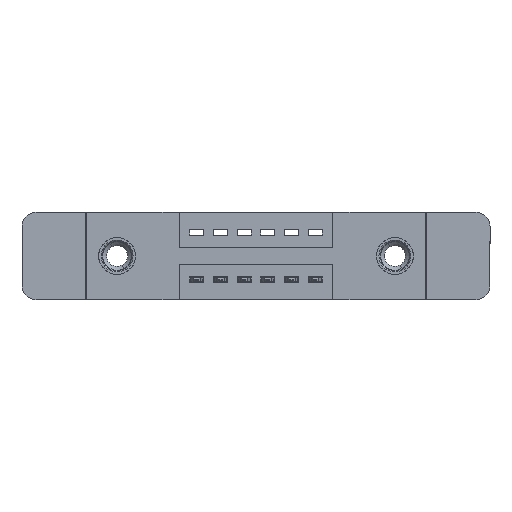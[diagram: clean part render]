
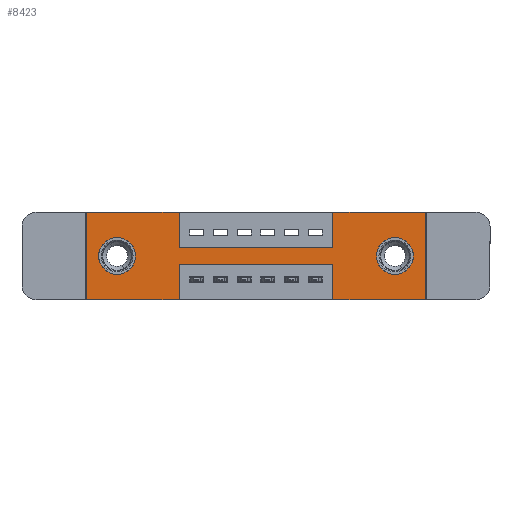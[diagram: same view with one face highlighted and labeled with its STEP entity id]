
A CAD part, front view. The second image highlights one B-rep face of the part: STEP entity #8423.
In plain terms, the highlighted planar face has unit normal (0, -1, 0).
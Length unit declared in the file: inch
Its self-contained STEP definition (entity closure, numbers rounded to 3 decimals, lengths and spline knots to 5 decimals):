
#94 = VERTEX_POINT ( 'NONE', #1673 ) ;
#147 = VERTEX_POINT ( 'NONE', #4214 ) ;
#158 = LINE ( 'NONE', #1594, #10441 ) ;
#370 = CARTESIAN_POINT ( 'NONE',  ( 1.305, 0., -0.185 ) ) ;
#415 = EDGE_CURVE ( 'NONE', #94, #5725, #7992, .T. ) ;
#497 = EDGE_LOOP ( 'NONE', ( #1147, #8711 ) ) ;
#560 = DIRECTION ( 'NONE',  ( 0., 0., -1. ) ) ;
#591 = DIRECTION ( 'NONE',  ( 0., 0., -1. ) ) ;
#706 = EDGE_CURVE ( 'NONE', #5725, #1700, #8682, .T. ) ;
#712 = PLANE ( 'NONE',  #7056 ) ;
#875 = VERTEX_POINT ( 'NONE', #2429 ) ;
#1141 = EDGE_CURVE ( 'NONE', #4067, #6682, #10605, .T. ) ;
#1147 = ORIENTED_EDGE ( 'NONE', *, *, #10740, .T. ) ;
#1435 = LINE ( 'NONE', #14208, #4059 ) ;
#1502 = ORIENTED_EDGE ( 'NONE', *, *, #9328, .F. ) ;
#1551 = DIRECTION ( 'NONE',  ( 0., 0., -1. ) ) ;
#1594 = CARTESIAN_POINT ( 'NONE',  ( 0.3925, 0., 0. ) ) ;
#1625 = EDGE_LOOP ( 'NONE', ( #4942, #13514, #14513, #9160, #2461, #1502, #2628, #13078, #1680, #3032, #5170, #10552 ) ) ;
#1673 = CARTESIAN_POINT ( 'NONE',  ( 1.435, 0., 0. ) ) ;
#1680 = ORIENTED_EDGE ( 'NONE', *, *, #2810, .F. ) ;
#1700 = VERTEX_POINT ( 'NONE', #3215 ) ;
#2200 = VERTEX_POINT ( 'NONE', #8379 ) ;
#2230 = EDGE_CURVE ( 'NONE', #14112, #12420, #10853, .T. ) ;
#2241 = DIRECTION ( 'NONE',  ( -1., 0., 0. ) ) ;
#2372 = AXIS2_PLACEMENT_3D ( 'NONE', #2486, #11525, #8225 ) ;
#2402 = EDGE_LOOP ( 'NONE', ( #5447, #10381 ) ) ;
#2429 = CARTESIAN_POINT ( 'NONE',  ( 0.13, 0., -0.107 ) ) ;
#2461 = ORIENTED_EDGE ( 'NONE', *, *, #415, .F. ) ;
#2466 = LINE ( 'NONE', #12484, #8844 ) ;
#2486 = CARTESIAN_POINT ( 'NONE',  ( 0.13, 0., -0.185 ) ) ;
#2627 = DIRECTION ( 'NONE',  ( 0., 0., -1. ) ) ;
#2628 = ORIENTED_EDGE ( 'NONE', *, *, #3161, .F. ) ;
#2651 = DIRECTION ( 'NONE',  ( -1., 0., 0. ) ) ;
#2701 = VERTEX_POINT ( 'NONE', #5728 ) ;
#2810 = EDGE_CURVE ( 'NONE', #6682, #5555, #158, .T. ) ;
#3032 = ORIENTED_EDGE ( 'NONE', *, *, #1141, .F. ) ;
#3161 = EDGE_CURVE ( 'NONE', #147, #13618, #6078, .T. ) ;
#3215 = CARTESIAN_POINT ( 'NONE',  ( 1.0425, 0., -0.37 ) ) ;
#3290 = AXIS2_PLACEMENT_3D ( 'NONE', #6904, #9589, #4974 ) ;
#3396 = VECTOR ( 'NONE', #10511, 39.37008 ) ;
#3418 = EDGE_CURVE ( 'NONE', #14611, #11170, #12412, .T. ) ;
#3650 = VECTOR ( 'NONE', #12302, 39.37008 ) ;
#4014 = LINE ( 'NONE', #13456, #3650 ) ;
#4059 = VECTOR ( 'NONE', #10851, 39.37008 ) ;
#4067 = VERTEX_POINT ( 'NONE', #6693 ) ;
#4214 = CARTESIAN_POINT ( 'NONE',  ( 1.0425, 0., -0.15 ) ) ;
#4367 = CARTESIAN_POINT ( 'NONE',  ( 0.3925, 0., -0.37 ) ) ;
#4815 = LINE ( 'NONE', #4888, #3396 ) ;
#4839 = CARTESIAN_POINT ( 'NONE',  ( 0., 0., 0. ) ) ;
#4888 = CARTESIAN_POINT ( 'NONE',  ( 1.0425, 0., -0.37 ) ) ;
#4942 = ORIENTED_EDGE ( 'NONE', *, *, #3418, .F. ) ;
#4974 = DIRECTION ( 'NONE',  ( 0., 0., 1. ) ) ;
#5170 = ORIENTED_EDGE ( 'NONE', *, *, #11163, .F. ) ;
#5447 = ORIENTED_EDGE ( 'NONE', *, *, #6535, .T. ) ;
#5555 = VERTEX_POINT ( 'NONE', #8791 ) ;
#5648 = VECTOR ( 'NONE', #8760, 39.37008 ) ;
#5725 = VERTEX_POINT ( 'NONE', #10052 ) ;
#5728 = CARTESIAN_POINT ( 'NONE',  ( 0., 0., -0.37 ) ) ;
#5973 = DIRECTION ( 'NONE',  ( 1., 0., 0. ) ) ;
#6078 = LINE ( 'NONE', #8991, #11801 ) ;
#6445 = CARTESIAN_POINT ( 'NONE',  ( 0., 0., -0.37 ) ) ;
#6506 = AXIS2_PLACEMENT_3D ( 'NONE', #370, #7164, #1551 ) ;
#6535 = EDGE_CURVE ( 'NONE', #12420, #14112, #7848, .T. ) ;
#6612 = CARTESIAN_POINT ( 'NONE',  ( 0.3925, 0., -0.37 ) ) ;
#6682 = VERTEX_POINT ( 'NONE', #11733 ) ;
#6693 = CARTESIAN_POINT ( 'NONE',  ( 0., 0., 0. ) ) ;
#6904 = CARTESIAN_POINT ( 'NONE',  ( 0.13, 0., -0.185 ) ) ;
#7056 = AXIS2_PLACEMENT_3D ( 'NONE', #7478, #7383, #560 ) ;
#7129 = CARTESIAN_POINT ( 'NONE',  ( 1.305, 0., -0.185 ) ) ;
#7164 = DIRECTION ( 'NONE',  ( 0., 1., 0. ) ) ;
#7276 = FACE_BOUND ( 'NONE', #497, .T. ) ;
#7383 = DIRECTION ( 'NONE',  ( 0., -1., 0. ) ) ;
#7478 = CARTESIAN_POINT ( 'NONE',  ( 0., 0., -0.37 ) ) ;
#7632 = FACE_OUTER_BOUND ( 'NONE', #1625, .T. ) ;
#7716 = DIRECTION ( 'NONE',  ( 0., 0., -1. ) ) ;
#7807 = CARTESIAN_POINT ( 'NONE',  ( 1.0425, 0., -0.22 ) ) ;
#7848 = CIRCLE ( 'NONE', #6506, 0.078 ) ;
#7936 = VECTOR ( 'NONE', #2651, 39.37008 ) ;
#7970 = FACE_BOUND ( 'NONE', #2402, .T. ) ;
#7992 = LINE ( 'NONE', #8221, #8351 ) ;
#8221 = CARTESIAN_POINT ( 'NONE',  ( 1.435, 0., 0. ) ) ;
#8225 = DIRECTION ( 'NONE',  ( 0., 0., 1. ) ) ;
#8262 = DIRECTION ( 'NONE',  ( 1., 0., 0. ) ) ;
#8351 = VECTOR ( 'NONE', #2627, 39.37008 ) ;
#8379 = CARTESIAN_POINT ( 'NONE',  ( 0.13, 0., -0.263 ) ) ;
#8387 = CIRCLE ( 'NONE', #2372, 0.078 ) ;
#8423 = ADVANCED_FACE ( 'NONE', ( #7970, #7276, #7632 ), #712, .T. ) ;
#8682 = LINE ( 'NONE', #6445, #5648 ) ;
#8711 = ORIENTED_EDGE ( 'NONE', *, *, #13481, .T. ) ;
#8760 = DIRECTION ( 'NONE',  ( -1., 0., 0. ) ) ;
#8791 = CARTESIAN_POINT ( 'NONE',  ( 0.3925, 0., -0.15 ) ) ;
#8802 = VECTOR ( 'NONE', #8262, 39.37008 ) ;
#8844 = VECTOR ( 'NONE', #5973, 39.37008 ) ;
#8991 = CARTESIAN_POINT ( 'NONE',  ( 1.0425, 0., 0. ) ) ;
#9091 = DIRECTION ( 'NONE',  ( 0., 0., 1. ) ) ;
#9096 = AXIS2_PLACEMENT_3D ( 'NONE', #7129, #9419, #10636 ) ;
#9148 = EDGE_CURVE ( 'NONE', #5555, #147, #1435, .T. ) ;
#9160 = ORIENTED_EDGE ( 'NONE', *, *, #706, .F. ) ;
#9328 = EDGE_CURVE ( 'NONE', #13618, #94, #2466, .T. ) ;
#9348 = CIRCLE ( 'NONE', #3290, 0.078 ) ;
#9419 = DIRECTION ( 'NONE',  ( 0., 1., 0. ) ) ;
#9589 = DIRECTION ( 'NONE',  ( 0., 1., 0. ) ) ;
#10052 = CARTESIAN_POINT ( 'NONE',  ( 1.435, 0., -0.37 ) ) ;
#10260 = CARTESIAN_POINT ( 'NONE',  ( 0.3925, 0., -0.22 ) ) ;
#10335 = VECTOR ( 'NONE', #2241, 39.37008 ) ;
#10353 = VERTEX_POINT ( 'NONE', #7807 ) ;
#10381 = ORIENTED_EDGE ( 'NONE', *, *, #2230, .T. ) ;
#10441 = VECTOR ( 'NONE', #591, 39.37008 ) ;
#10511 = DIRECTION ( 'NONE',  ( 0., 0., 1. ) ) ;
#10552 = ORIENTED_EDGE ( 'NONE', *, *, #10588, .F. ) ;
#10588 = EDGE_CURVE ( 'NONE', #11170, #2701, #13285, .T. ) ;
#10605 = LINE ( 'NONE', #4839, #8802 ) ;
#10636 = DIRECTION ( 'NONE',  ( 0., 0., -1. ) ) ;
#10740 = EDGE_CURVE ( 'NONE', #875, #2200, #9348, .T. ) ;
#10851 = DIRECTION ( 'NONE',  ( 1., 0., 0. ) ) ;
#10853 = CIRCLE ( 'NONE', #9096, 0.078 ) ;
#11163 = EDGE_CURVE ( 'NONE', #2701, #4067, #4014, .T. ) ;
#11170 = VERTEX_POINT ( 'NONE', #6612 ) ;
#11403 = CARTESIAN_POINT ( 'NONE',  ( 0.3925, 0., -0.22 ) ) ;
#11525 = DIRECTION ( 'NONE',  ( 0., 1., 0. ) ) ;
#11679 = VECTOR ( 'NONE', #7716, 39.37008 ) ;
#11733 = CARTESIAN_POINT ( 'NONE',  ( 0.3925, 0., 0. ) ) ;
#11771 = CARTESIAN_POINT ( 'NONE',  ( 1.305, 0., -0.107 ) ) ;
#11801 = VECTOR ( 'NONE', #9091, 39.37008 ) ;
#12302 = DIRECTION ( 'NONE',  ( 0., 0., 1. ) ) ;
#12412 = LINE ( 'NONE', #4367, #11679 ) ;
#12420 = VERTEX_POINT ( 'NONE', #11771 ) ;
#12484 = CARTESIAN_POINT ( 'NONE',  ( 0., 0., 0. ) ) ;
#12740 = CARTESIAN_POINT ( 'NONE',  ( 0., 0., -0.37 ) ) ;
#12905 = CARTESIAN_POINT ( 'NONE',  ( 1.305, 0., -0.263 ) ) ;
#13078 = ORIENTED_EDGE ( 'NONE', *, *, #9148, .F. ) ;
#13175 = LINE ( 'NONE', #10260, #10335 ) ;
#13285 = LINE ( 'NONE', #12740, #7936 ) ;
#13456 = CARTESIAN_POINT ( 'NONE',  ( 0., 0., 0. ) ) ;
#13481 = EDGE_CURVE ( 'NONE', #2200, #875, #8387, .T. ) ;
#13514 = ORIENTED_EDGE ( 'NONE', *, *, #13955, .F. ) ;
#13618 = VERTEX_POINT ( 'NONE', #14155 ) ;
#13955 = EDGE_CURVE ( 'NONE', #10353, #14611, #13175, .T. ) ;
#13983 = EDGE_CURVE ( 'NONE', #1700, #10353, #4815, .T. ) ;
#14112 = VERTEX_POINT ( 'NONE', #12905 ) ;
#14155 = CARTESIAN_POINT ( 'NONE',  ( 1.0425, 0., 0. ) ) ;
#14208 = CARTESIAN_POINT ( 'NONE',  ( 0.3925, 0., -0.15 ) ) ;
#14513 = ORIENTED_EDGE ( 'NONE', *, *, #13983, .F. ) ;
#14611 = VERTEX_POINT ( 'NONE', #11403 ) ;
